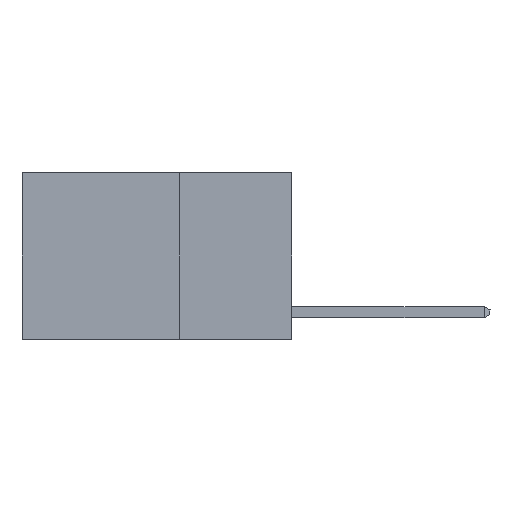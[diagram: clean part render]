
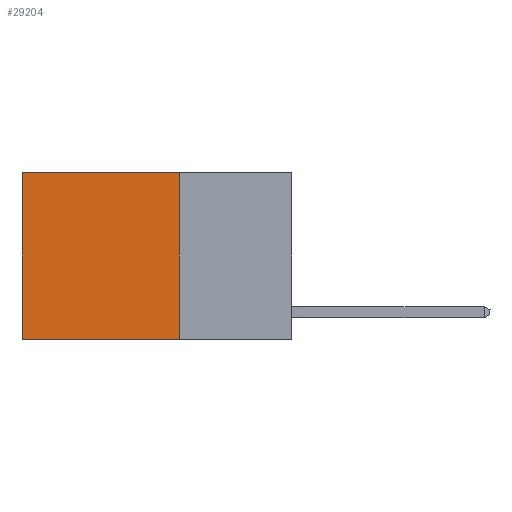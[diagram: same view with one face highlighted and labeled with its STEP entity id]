
A CAD part, left-side view. The second image highlights one B-rep face of the part: STEP entity #29204.
In plain terms, the highlighted planar face has unit normal (-1, 0, 0).
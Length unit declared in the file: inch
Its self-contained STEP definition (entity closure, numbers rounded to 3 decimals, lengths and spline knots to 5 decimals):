
#574 = DIRECTION ( 'NONE',  ( 0., 0., -1. ) ) ;
#2260 = LINE ( 'NONE', #5902, #20888 ) ;
#2894 = DIRECTION ( 'NONE',  ( 0., 0., -1. ) ) ;
#3041 = VERTEX_POINT ( 'NONE', #17168 ) ;
#5902 = CARTESIAN_POINT ( 'NONE',  ( 0.2625, 0.25, 0. ) ) ;
#6453 = ORIENTED_EDGE ( 'NONE', *, *, #27703, .F. ) ;
#8457 = CARTESIAN_POINT ( 'NONE',  ( 0.2625, 0.25, 0. ) ) ;
#8752 = AXIS2_PLACEMENT_3D ( 'NONE', #8967, #26262, #2894 ) ;
#8967 = CARTESIAN_POINT ( 'NONE',  ( 0.2625, 0.25, 0. ) ) ;
#10916 = LINE ( 'NONE', #12133, #14928 ) ;
#11863 = CARTESIAN_POINT ( 'NONE',  ( 0.2625, 0.25, -0.37 ) ) ;
#12133 = CARTESIAN_POINT ( 'NONE',  ( 0.2625, 0.6, 0. ) ) ;
#12748 = CARTESIAN_POINT ( 'NONE',  ( 0.2625, 0.6, 0. ) ) ;
#13983 = FACE_OUTER_BOUND ( 'NONE', #29916, .T. ) ;
#14089 = VERTEX_POINT ( 'NONE', #20513 ) ;
#14094 = VECTOR ( 'NONE', #25981, 39.37008 ) ;
#14928 = VECTOR ( 'NONE', #574, 39.37008 ) ;
#15190 = VECTOR ( 'NONE', #25196, 39.37008 ) ;
#15506 = VERTEX_POINT ( 'NONE', #11863 ) ;
#15622 = ORIENTED_EDGE ( 'NONE', *, *, #23891, .T. ) ;
#17168 = CARTESIAN_POINT ( 'NONE',  ( 0.2625, 0.25, 0. ) ) ;
#20350 = EDGE_CURVE ( 'NONE', #15506, #14089, #25052, .T. ) ;
#20362 = LINE ( 'NONE', #8457, #14094 ) ;
#20513 = CARTESIAN_POINT ( 'NONE',  ( 0.2625, 0.6, -0.37 ) ) ;
#20888 = VECTOR ( 'NONE', #22213, 39.37008 ) ;
#22016 = ORIENTED_EDGE ( 'NONE', *, *, #22576, .T. ) ;
#22213 = DIRECTION ( 'NONE',  ( 0., 1., 0. ) ) ;
#22576 = EDGE_CURVE ( 'NONE', #3041, #23212, #2260, .T. ) ;
#22876 = PLANE ( 'NONE',  #8752 ) ;
#23212 = VERTEX_POINT ( 'NONE', #12748 ) ;
#23891 = EDGE_CURVE ( 'NONE', #23212, #14089, #10916, .T. ) ;
#25052 = LINE ( 'NONE', #27434, #15190 ) ;
#25196 = DIRECTION ( 'NONE',  ( 0., 1., 0. ) ) ;
#25981 = DIRECTION ( 'NONE',  ( 0., 0., -1. ) ) ;
#26262 = DIRECTION ( 'NONE',  ( 1., 0., 0. ) ) ;
#27434 = CARTESIAN_POINT ( 'NONE',  ( 0.2625, 0.25, -0.37 ) ) ;
#27703 = EDGE_CURVE ( 'NONE', #3041, #15506, #20362, .T. ) ;
#28412 = ORIENTED_EDGE ( 'NONE', *, *, #20350, .F. ) ;
#29204 = ADVANCED_FACE ( 'NONE', ( #13983 ), #22876, .F. ) ;
#29916 = EDGE_LOOP ( 'NONE', ( #15622, #28412, #6453, #22016 ) ) ;
